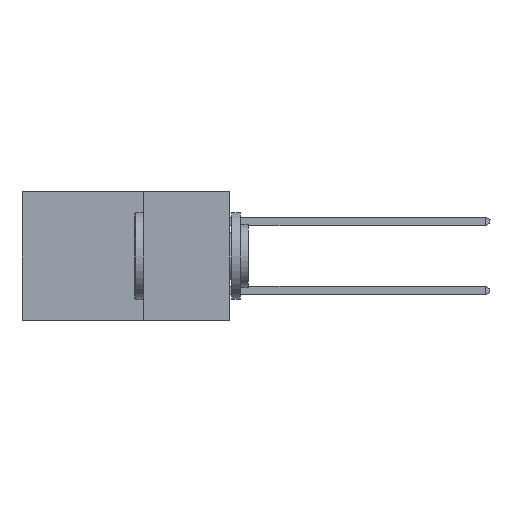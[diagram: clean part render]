
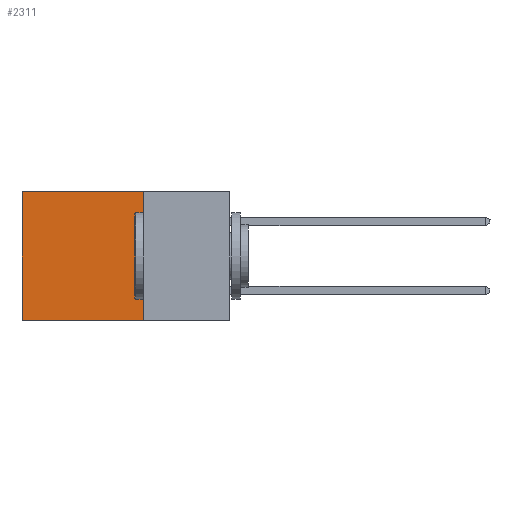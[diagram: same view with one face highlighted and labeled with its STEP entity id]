
A CAD part, left-side view. The second image highlights one B-rep face of the part: STEP entity #2311.
In plain terms, the highlighted planar face has unit normal (-1, 0, 0).
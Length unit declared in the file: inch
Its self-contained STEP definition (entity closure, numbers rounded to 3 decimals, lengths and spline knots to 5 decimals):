
#2167 = CARTESIAN_POINT ( 'NONE',  ( 0.2615, 0.25, -0.37 ) ) ;
#2311 = ADVANCED_FACE ( 'NONE', ( #21348 ), #23504, .F. ) ;
#2405 = DIRECTION ( 'NONE',  ( 0., 0., -1. ) ) ;
#2437 = DIRECTION ( 'NONE',  ( 0., 1., 0. ) ) ;
#2688 = AXIS2_PLACEMENT_3D ( 'NONE', #2167, #10257, #2405 ) ;
#4245 = DIRECTION ( 'NONE',  ( 0., 0., -1. ) ) ;
#4857 = VECTOR ( 'NONE', #2437, 39.37008 ) ;
#5731 = EDGE_CURVE ( 'NONE', #13097, #10878, #8523, .T. ) ;
#6110 = ORIENTED_EDGE ( 'NONE', *, *, #14799, .T. ) ;
#6363 = CARTESIAN_POINT ( 'NONE',  ( 0.2615, 0.25, -0.37 ) ) ;
#6391 = VECTOR ( 'NONE', #4245, 39.37008 ) ;
#6917 = VECTOR ( 'NONE', #20004, 39.37008 ) ;
#7533 = EDGE_LOOP ( 'NONE', ( #6110, #15726, #18806, #9020 ) ) ;
#7895 = CARTESIAN_POINT ( 'NONE',  ( 0.2615, 0.6, -0.37 ) ) ;
#8523 = LINE ( 'NONE', #16463, #6917 ) ;
#9020 = ORIENTED_EDGE ( 'NONE', *, *, #10302, .T. ) ;
#10257 = DIRECTION ( 'NONE',  ( 1., 0., 0. ) ) ;
#10302 = EDGE_CURVE ( 'NONE', #13097, #21369, #14085, .T. ) ;
#10679 = CARTESIAN_POINT ( 'NONE',  ( 0.2615, 0.25, 0. ) ) ;
#10878 = VERTEX_POINT ( 'NONE', #24777 ) ;
#13097 = VERTEX_POINT ( 'NONE', #22258 ) ;
#13577 = LINE ( 'NONE', #7895, #6391 ) ;
#14085 = LINE ( 'NONE', #10679, #24576 ) ;
#14799 = EDGE_CURVE ( 'NONE', #21369, #18253, #13577, .T. ) ;
#14837 = CARTESIAN_POINT ( 'NONE',  ( 0.2615, 0.6, 0. ) ) ;
#15726 = ORIENTED_EDGE ( 'NONE', *, *, #17180, .F. ) ;
#16357 = DIRECTION ( 'NONE',  ( 0., 1., 0. ) ) ;
#16463 = CARTESIAN_POINT ( 'NONE',  ( 0.2615, 0.25, -0.37 ) ) ;
#17180 = EDGE_CURVE ( 'NONE', #10878, #18253, #19753, .T. ) ;
#18253 = VERTEX_POINT ( 'NONE', #20315 ) ;
#18806 = ORIENTED_EDGE ( 'NONE', *, *, #5731, .F. ) ;
#19753 = LINE ( 'NONE', #6363, #4857 ) ;
#20004 = DIRECTION ( 'NONE',  ( 0., 0., -1. ) ) ;
#20315 = CARTESIAN_POINT ( 'NONE',  ( 0.2615, 0.6, -0.37 ) ) ;
#21348 = FACE_OUTER_BOUND ( 'NONE', #7533, .T. ) ;
#21369 = VERTEX_POINT ( 'NONE', #14837 ) ;
#22258 = CARTESIAN_POINT ( 'NONE',  ( 0.2615, 0.25, 0. ) ) ;
#23504 = PLANE ( 'NONE',  #2688 ) ;
#24576 = VECTOR ( 'NONE', #16357, 39.37008 ) ;
#24777 = CARTESIAN_POINT ( 'NONE',  ( 0.2615, 0.25, -0.37 ) ) ;
